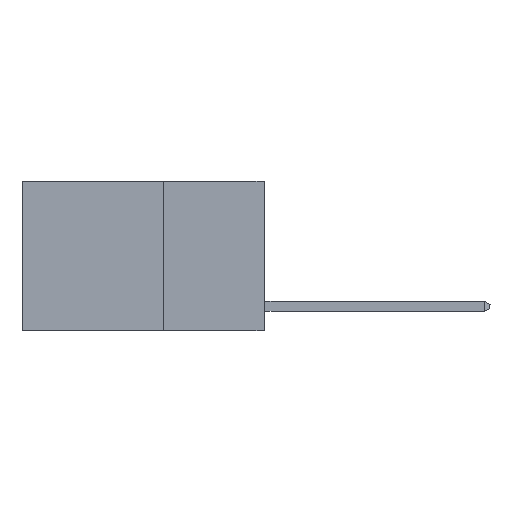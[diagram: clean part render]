
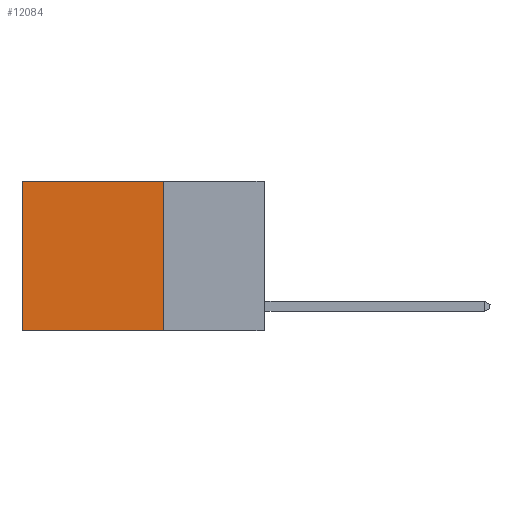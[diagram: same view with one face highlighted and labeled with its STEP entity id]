
A CAD part, left-side view. The second image highlights one B-rep face of the part: STEP entity #12084.
In plain terms, the highlighted planar face has unit normal (-1, 0, 0).
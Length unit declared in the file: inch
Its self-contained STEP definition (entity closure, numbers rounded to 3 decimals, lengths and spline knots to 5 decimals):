
#707 = DIRECTION ( 'NONE',  ( 0., 1., 0. ) ) ;
#824 = LINE ( 'NONE', #16059, #8994 ) ;
#1331 = LINE ( 'NONE', #20357, #17740 ) ;
#1743 = VERTEX_POINT ( 'NONE', #14016 ) ;
#2332 = ORIENTED_EDGE ( 'NONE', *, *, #17093, .F. ) ;
#2525 = DIRECTION ( 'NONE',  ( 0., 0., -1. ) ) ;
#3071 = DIRECTION ( 'NONE',  ( 0., 0., -1. ) ) ;
#4394 = CARTESIAN_POINT ( 'NONE',  ( 0.2625, 0.6, -0.37 ) ) ;
#5339 = LINE ( 'NONE', #20866, #18439 ) ;
#5941 = EDGE_CURVE ( 'NONE', #16131, #19967, #824, .T. ) ;
#6352 = EDGE_CURVE ( 'NONE', #13931, #1743, #1331, .T. ) ;
#8994 = VECTOR ( 'NONE', #17721, 39.37008 ) ;
#9116 = CARTESIAN_POINT ( 'NONE',  ( 0.2625, 0.6, 0. ) ) ;
#9313 = CARTESIAN_POINT ( 'NONE',  ( 0.2625, 0.25, -0.37 ) ) ;
#9994 = ORIENTED_EDGE ( 'NONE', *, *, #5941, .F. ) ;
#11083 = DIRECTION ( 'NONE',  ( 0., 0., -1. ) ) ;
#11209 = CARTESIAN_POINT ( 'NONE',  ( 0.2625, 0.25, 0. ) ) ;
#11287 = PLANE ( 'NONE',  #18206 ) ;
#11959 = ORIENTED_EDGE ( 'NONE', *, *, #6352, .T. ) ;
#12084 = ADVANCED_FACE ( 'NONE', ( #20842 ), #11287, .F. ) ;
#12138 = LINE ( 'NONE', #9116, #15943 ) ;
#12926 = DIRECTION ( 'NONE',  ( 1., 0., 0. ) ) ;
#12982 = EDGE_LOOP ( 'NONE', ( #19502, #9994, #2332, #11959 ) ) ;
#13931 = VERTEX_POINT ( 'NONE', #11209 ) ;
#14016 = CARTESIAN_POINT ( 'NONE',  ( 0.2625, 0.6, 0. ) ) ;
#15943 = VECTOR ( 'NONE', #2525, 39.37008 ) ;
#16059 = CARTESIAN_POINT ( 'NONE',  ( 0.2625, 0.25, -0.37 ) ) ;
#16131 = VERTEX_POINT ( 'NONE', #9313 ) ;
#17093 = EDGE_CURVE ( 'NONE', #13931, #16131, #5339, .T. ) ;
#17721 = DIRECTION ( 'NONE',  ( 0., 1., 0. ) ) ;
#17740 = VECTOR ( 'NONE', #707, 39.37008 ) ;
#18206 = AXIS2_PLACEMENT_3D ( 'NONE', #21059, #12926, #3071 ) ;
#18439 = VECTOR ( 'NONE', #11083, 39.37008 ) ;
#19502 = ORIENTED_EDGE ( 'NONE', *, *, #20367, .T. ) ;
#19967 = VERTEX_POINT ( 'NONE', #4394 ) ;
#20357 = CARTESIAN_POINT ( 'NONE',  ( 0.2625, 0.25, 0. ) ) ;
#20367 = EDGE_CURVE ( 'NONE', #1743, #19967, #12138, .T. ) ;
#20842 = FACE_OUTER_BOUND ( 'NONE', #12982, .T. ) ;
#20866 = CARTESIAN_POINT ( 'NONE',  ( 0.2625, 0.25, 0. ) ) ;
#21059 = CARTESIAN_POINT ( 'NONE',  ( 0.2625, 0.25, 0. ) ) ;
